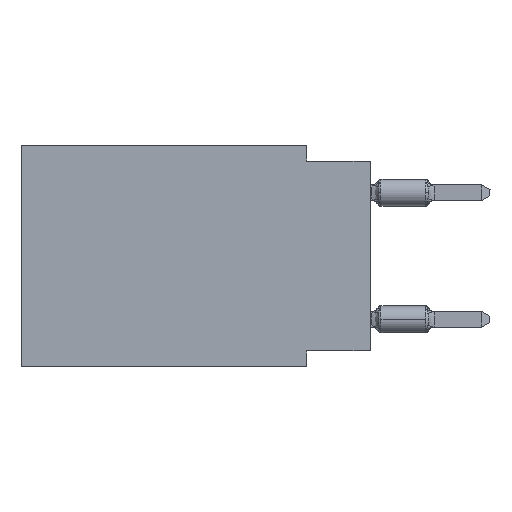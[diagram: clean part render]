
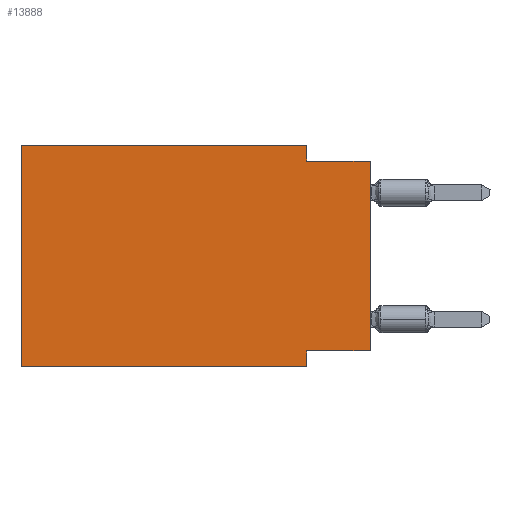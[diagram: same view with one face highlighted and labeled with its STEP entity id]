
A CAD part, left-side view. The second image highlights one B-rep face of the part: STEP entity #13888.
In plain terms, the highlighted planar face has unit normal (-1, 0, 0).
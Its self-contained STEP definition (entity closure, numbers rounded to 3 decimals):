
#588 = PLANE ( 'NONE',  #16887 ) ;
#1032 = LINE ( 'NONE', #10913, #1149 ) ;
#1149 = VECTOR ( 'NONE', #19059, 1000. ) ;
#1489 = VERTEX_POINT ( 'NONE', #16809 ) ;
#1589 = CARTESIAN_POINT ( 'NONE',  ( 0., 2.54, -8.89 ) ) ;
#2010 = DIRECTION ( 'NONE',  ( 0., 0., -1. ) ) ;
#2396 = DIRECTION ( 'NONE',  ( 0., 0., -1. ) ) ;
#2591 = LINE ( 'NONE', #4125, #18297 ) ;
#3200 = EDGE_CURVE ( 'NONE', #6187, #3860, #9746, .T. ) ;
#3344 = LINE ( 'NONE', #17997, #21311 ) ;
#3361 = VERTEX_POINT ( 'NONE', #11016 ) ;
#3860 = VERTEX_POINT ( 'NONE', #11653 ) ;
#4125 = CARTESIAN_POINT ( 'NONE',  ( 0., 13.97, 0. ) ) ;
#4406 = ORIENTED_EDGE ( 'NONE', *, *, #9919, .T. ) ;
#4433 = LINE ( 'NONE', #1589, #4886 ) ;
#4886 = VECTOR ( 'NONE', #11361, 1000. ) ;
#4988 = CARTESIAN_POINT ( 'NONE',  ( 0., 0., -0.635 ) ) ;
#5712 = EDGE_CURVE ( 'NONE', #16774, #19203, #2591, .T. ) ;
#6187 = VERTEX_POINT ( 'NONE', #15697 ) ;
#6502 = CARTESIAN_POINT ( 'NONE',  ( 0., 2.54, 0. ) ) ;
#6557 = CARTESIAN_POINT ( 'NONE',  ( 0., 0., -8.255 ) ) ;
#7281 = LINE ( 'NONE', #9119, #14265 ) ;
#7702 = CARTESIAN_POINT ( 'NONE',  ( 0., 0., -8.255 ) ) ;
#8383 = ORIENTED_EDGE ( 'NONE', *, *, #16481, .F. ) ;
#8479 = EDGE_CURVE ( 'NONE', #19203, #9669, #3344, .T. ) ;
#8669 = CARTESIAN_POINT ( 'NONE',  ( 0., 13.97, 0. ) ) ;
#9119 = CARTESIAN_POINT ( 'NONE',  ( 0., 2.54, 0. ) ) ;
#9588 = LINE ( 'NONE', #6557, #18381 ) ;
#9669 = VERTEX_POINT ( 'NONE', #6502 ) ;
#9746 = LINE ( 'NONE', #4988, #13005 ) ;
#9919 = EDGE_CURVE ( 'NONE', #13350, #3860, #1032, .T. ) ;
#10850 = LINE ( 'NONE', #19334, #15642 ) ;
#10913 = CARTESIAN_POINT ( 'NONE',  ( 0., 0., 0. ) ) ;
#11016 = CARTESIAN_POINT ( 'NONE',  ( 0., 2.54, -8.89 ) ) ;
#11361 = DIRECTION ( 'NONE',  ( 0., 0., -1. ) ) ;
#11593 = DIRECTION ( 'NONE',  ( 0., -1., 0. ) ) ;
#11653 = CARTESIAN_POINT ( 'NONE',  ( 0., 0., -0.635 ) ) ;
#11823 = ORIENTED_EDGE ( 'NONE', *, *, #20484, .F. ) ;
#12935 = ORIENTED_EDGE ( 'NONE', *, *, #3200, .F. ) ;
#13005 = VECTOR ( 'NONE', #11593, 1000. ) ;
#13350 = VERTEX_POINT ( 'NONE', #7702 ) ;
#13670 = ORIENTED_EDGE ( 'NONE', *, *, #5712, .F. ) ;
#13888 = ADVANCED_FACE ( 'NONE', ( #15167 ), #588, .F. ) ;
#14265 = VECTOR ( 'NONE', #2396, 1000. ) ;
#14968 = DIRECTION ( 'NONE',  ( 0., -1., 0. ) ) ;
#15167 = FACE_OUTER_BOUND ( 'NONE', #15570, .T. ) ;
#15283 = ORIENTED_EDGE ( 'NONE', *, *, #19024, .T. ) ;
#15570 = EDGE_LOOP ( 'NONE', ( #4406, #12935, #20414, #21203, #13670, #15283, #8383, #11823 ) ) ;
#15642 = VECTOR ( 'NONE', #17476, 1000. ) ;
#15697 = CARTESIAN_POINT ( 'NONE',  ( 0., 2.54, -0.635 ) ) ;
#15723 = DIRECTION ( 'NONE',  ( 0., 0., 1. ) ) ;
#16481 = EDGE_CURVE ( 'NONE', #1489, #3361, #4433, .T. ) ;
#16774 = VERTEX_POINT ( 'NONE', #20566 ) ;
#16809 = CARTESIAN_POINT ( 'NONE',  ( 0., 2.54, -8.255 ) ) ;
#16887 = AXIS2_PLACEMENT_3D ( 'NONE', #18724, #20460, #2010 ) ;
#17476 = DIRECTION ( 'NONE',  ( 0., -1., 0. ) ) ;
#17997 = CARTESIAN_POINT ( 'NONE',  ( 0., 13.97, 0. ) ) ;
#18297 = VECTOR ( 'NONE', #15723, 1000. ) ;
#18381 = VECTOR ( 'NONE', #19580, 1000. ) ;
#18724 = CARTESIAN_POINT ( 'NONE',  ( 0., 13.97, 0. ) ) ;
#18960 = EDGE_CURVE ( 'NONE', #9669, #6187, #7281, .T. ) ;
#19024 = EDGE_CURVE ( 'NONE', #16774, #3361, #10850, .T. ) ;
#19059 = DIRECTION ( 'NONE',  ( 0., 0., 1. ) ) ;
#19203 = VERTEX_POINT ( 'NONE', #8669 ) ;
#19334 = CARTESIAN_POINT ( 'NONE',  ( 0., 13.97, -8.89 ) ) ;
#19580 = DIRECTION ( 'NONE',  ( 0., 1., 0. ) ) ;
#20414 = ORIENTED_EDGE ( 'NONE', *, *, #18960, .F. ) ;
#20460 = DIRECTION ( 'NONE',  ( 1., 0., 0. ) ) ;
#20484 = EDGE_CURVE ( 'NONE', #13350, #1489, #9588, .T. ) ;
#20566 = CARTESIAN_POINT ( 'NONE',  ( 0., 13.97, -8.89 ) ) ;
#21203 = ORIENTED_EDGE ( 'NONE', *, *, #8479, .F. ) ;
#21311 = VECTOR ( 'NONE', #14968, 1000. ) ;
